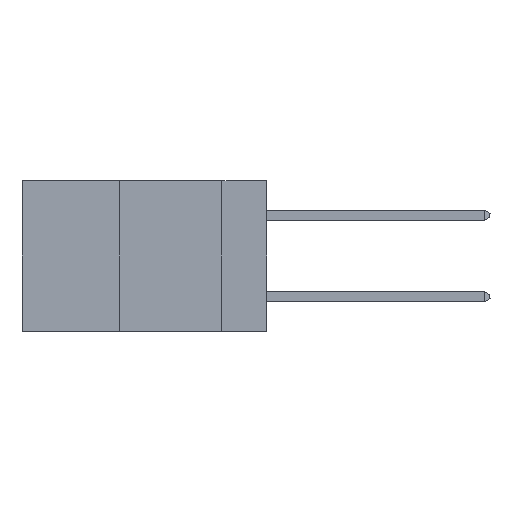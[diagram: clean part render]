
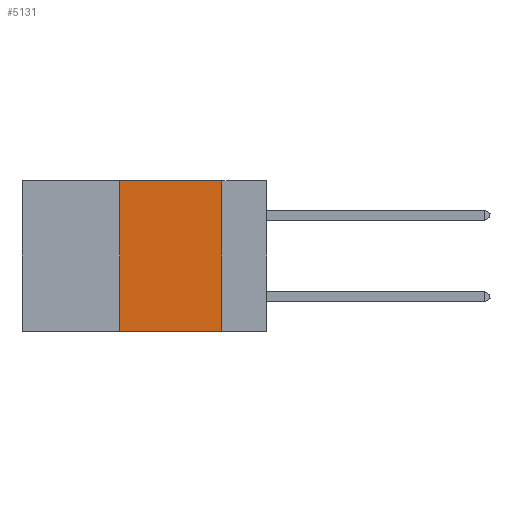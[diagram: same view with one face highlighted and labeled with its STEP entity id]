
A CAD part, left-side view. The second image highlights one B-rep face of the part: STEP entity #5131.
In plain terms, the highlighted planar face has unit normal (-1, 0, 0).
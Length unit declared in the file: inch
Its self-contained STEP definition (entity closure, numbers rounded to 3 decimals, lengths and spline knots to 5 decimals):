
#404 = VERTEX_POINT ( 'NONE', #11749 ) ;
#420 = VERTEX_POINT ( 'NONE', #11442 ) ;
#628 = CARTESIAN_POINT ( 'NONE',  ( 0., 0.11, 0. ) ) ;
#2299 = EDGE_CURVE ( 'NONE', #404, #10289, #5921, .T. ) ;
#2418 = VECTOR ( 'NONE', #9292, 39.37008 ) ;
#2705 = VECTOR ( 'NONE', #13249, 39.37008 ) ;
#3151 = ORIENTED_EDGE ( 'NONE', *, *, #7739, .F. ) ;
#4664 = AXIS2_PLACEMENT_3D ( 'NONE', #12331, #12352, #13259 ) ;
#4976 = ORIENTED_EDGE ( 'NONE', *, *, #2299, .F. ) ;
#5131 = ADVANCED_FACE ( 'NONE', ( #5259 ), #13246, .F. ) ;
#5259 = FACE_OUTER_BOUND ( 'NONE', #8781, .T. ) ;
#5314 = VERTEX_POINT ( 'NONE', #11320 ) ;
#5339 = LINE ( 'NONE', #628, #2418 ) ;
#5849 = CARTESIAN_POINT ( 'NONE',  ( 0., 0.6, -0.37 ) ) ;
#5921 = LINE ( 'NONE', #8283, #14962 ) ;
#5962 = CARTESIAN_POINT ( 'NONE',  ( 0., 0.36, 0. ) ) ;
#5996 = EDGE_CURVE ( 'NONE', #404, #420, #12350, .T. ) ;
#6898 = VECTOR ( 'NONE', #11960, 39.37008 ) ;
#7326 = ORIENTED_EDGE ( 'NONE', *, *, #8689, .F. ) ;
#7550 = DIRECTION ( 'NONE',  ( 0., 0., 1. ) ) ;
#7739 = EDGE_CURVE ( 'NONE', #5314, #420, #5339, .T. ) ;
#8283 = CARTESIAN_POINT ( 'NONE',  ( 0., 0.36, 0. ) ) ;
#8689 = EDGE_CURVE ( 'NONE', #10289, #5314, #13165, .T. ) ;
#8766 = ORIENTED_EDGE ( 'NONE', *, *, #5996, .T. ) ;
#8781 = EDGE_LOOP ( 'NONE', ( #3151, #7326, #4976, #8766 ) ) ;
#9292 = DIRECTION ( 'NONE',  ( 0., 0., -1. ) ) ;
#10289 = VERTEX_POINT ( 'NONE', #5962 ) ;
#11320 = CARTESIAN_POINT ( 'NONE',  ( 0., 0.11, 0. ) ) ;
#11442 = CARTESIAN_POINT ( 'NONE',  ( 0., 0.11, -0.37 ) ) ;
#11749 = CARTESIAN_POINT ( 'NONE',  ( 0., 0.36, -0.37 ) ) ;
#11960 = DIRECTION ( 'NONE',  ( 0., -1., 0. ) ) ;
#12331 = CARTESIAN_POINT ( 'NONE',  ( 0., 0.6, 0. ) ) ;
#12350 = LINE ( 'NONE', #5849, #2705 ) ;
#12352 = DIRECTION ( 'NONE',  ( 1., 0., 0. ) ) ;
#13149 = CARTESIAN_POINT ( 'NONE',  ( 0., 0.6, 0. ) ) ;
#13165 = LINE ( 'NONE', #13149, #6898 ) ;
#13246 = PLANE ( 'NONE',  #4664 ) ;
#13249 = DIRECTION ( 'NONE',  ( 0., -1., 0. ) ) ;
#13259 = DIRECTION ( 'NONE',  ( 0., 0., -1. ) ) ;
#14962 = VECTOR ( 'NONE', #7550, 39.37008 ) ;
